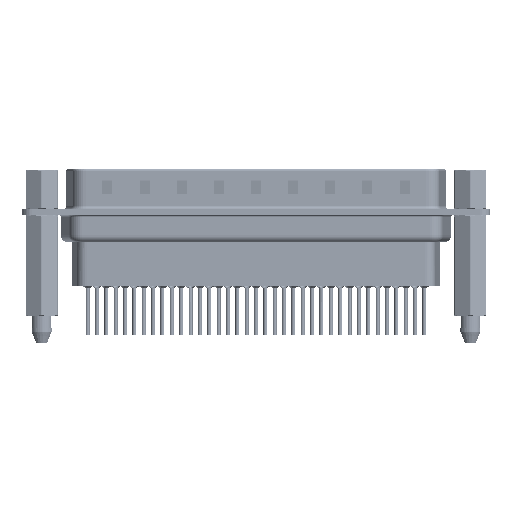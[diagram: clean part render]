
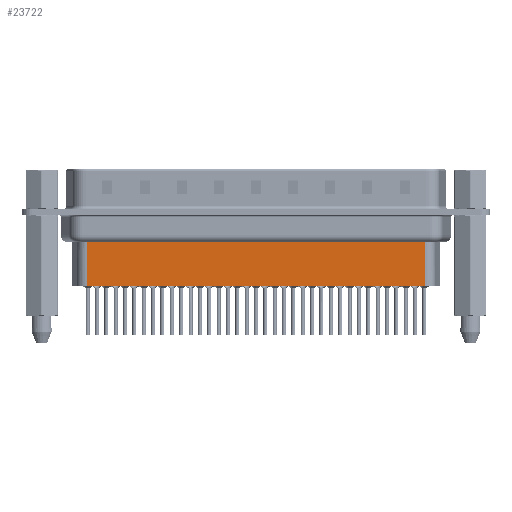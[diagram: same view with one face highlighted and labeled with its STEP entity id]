
A CAD part, front view. The second image highlights one B-rep face of the part: STEP entity #23722.
In plain terms, the highlighted planar face has unit normal (0, -1, 0).
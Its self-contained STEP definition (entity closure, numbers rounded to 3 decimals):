
#748 = CARTESIAN_POINT ( 'NONE',  ( 6.706, -3.5, -10.95 ) ) ;
#1562 = FACE_OUTER_BOUND ( 'NONE', #8497, .T. ) ;
#2368 = VECTOR ( 'NONE', #13283, 1000. ) ;
#4358 = DIRECTION ( 'NONE',  ( 0., -1., 0. ) ) ;
#4874 = CARTESIAN_POINT ( 'NONE',  ( 6.706, -3.5, -3.1 ) ) ;
#5671 = DIRECTION ( 'NONE',  ( -1., 0., 0. ) ) ;
#5688 = CARTESIAN_POINT ( 'NONE',  ( 6.706, -3.5, -10.95 ) ) ;
#5934 = VECTOR ( 'NONE', #5671, 1000. ) ;
#6797 = DIRECTION ( 'NONE',  ( 1., 0., 0. ) ) ;
#7541 = CARTESIAN_POINT ( 'NONE',  ( 56.794, -3.5, -4.097 ) ) ;
#8497 = EDGE_LOOP ( 'NONE', ( #34806, #35906, #9561, #22869 ) ) ;
#8866 = EDGE_CURVE ( 'NONE', #16152, #30185, #19888, .T. ) ;
#9561 = ORIENTED_EDGE ( 'NONE', *, *, #28143, .T. ) ;
#10074 = VERTEX_POINT ( 'NONE', #33701 ) ;
#13283 = DIRECTION ( 'NONE',  ( 0., 0., -1. ) ) ;
#14274 = DIRECTION ( 'NONE',  ( -1., 0., 0. ) ) ;
#16152 = VERTEX_POINT ( 'NONE', #7541 ) ;
#16485 = VECTOR ( 'NONE', #14274, 1000. ) ;
#18012 = CARTESIAN_POINT ( 'NONE',  ( 56.794, -3.5, -3.1 ) ) ;
#19888 = LINE ( 'NONE', #28891, #5934 ) ;
#19902 = EDGE_CURVE ( 'NONE', #16152, #10074, #26996, .T. ) ;
#22869 = ORIENTED_EDGE ( 'NONE', *, *, #23330, .F. ) ;
#23330 = EDGE_CURVE ( 'NONE', #10074, #25514, #31330, .T. ) ;
#23722 = ADVANCED_FACE ( 'NONE', ( #1562 ), #35800, .T. ) ;
#24176 = DIRECTION ( 'NONE',  ( 0., 0., -1. ) ) ;
#25514 = VERTEX_POINT ( 'NONE', #748 ) ;
#26996 = LINE ( 'NONE', #18012, #27292 ) ;
#27292 = VECTOR ( 'NONE', #24176, 1000. ) ;
#27350 = LINE ( 'NONE', #4874, #2368 ) ;
#28143 = EDGE_CURVE ( 'NONE', #30185, #25514, #27350, .T. ) ;
#28298 = CARTESIAN_POINT ( 'NONE',  ( 6.706, -3.5, -4.097 ) ) ;
#28891 = CARTESIAN_POINT ( 'NONE',  ( 6.459, -3.5, -4.097 ) ) ;
#30185 = VERTEX_POINT ( 'NONE', #28298 ) ;
#31330 = LINE ( 'NONE', #5688, #16485 ) ;
#33701 = CARTESIAN_POINT ( 'NONE',  ( 56.794, -3.5, -10.95 ) ) ;
#34806 = ORIENTED_EDGE ( 'NONE', *, *, #19902, .F. ) ;
#35246 = CARTESIAN_POINT ( 'NONE',  ( 6.706, -3.5, -3.1 ) ) ;
#35637 = AXIS2_PLACEMENT_3D ( 'NONE', #35246, #4358, #6797 ) ;
#35800 = PLANE ( 'NONE',  #35637 ) ;
#35906 = ORIENTED_EDGE ( 'NONE', *, *, #8866, .T. ) ;
